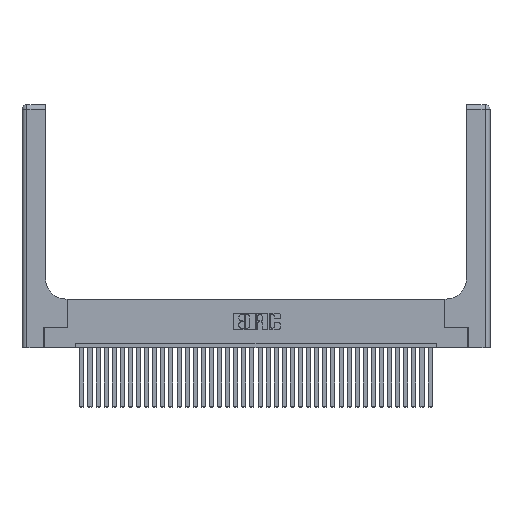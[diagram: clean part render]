
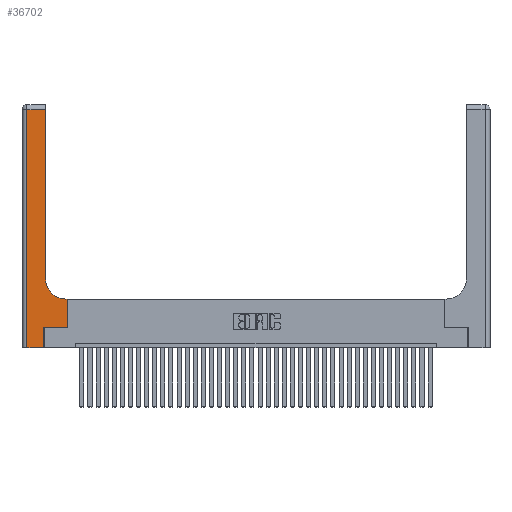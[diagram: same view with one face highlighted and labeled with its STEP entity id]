
A CAD part, top view. The second image highlights one B-rep face of the part: STEP entity #36702.
In plain terms, the highlighted planar face has unit normal (0, 0, 1).
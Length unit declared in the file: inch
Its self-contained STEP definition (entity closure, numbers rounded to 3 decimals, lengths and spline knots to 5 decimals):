
#1212 = EDGE_CURVE ( 'NONE', #21255, #14753, #31797, .T. ) ;
#1255 = ORIENTED_EDGE ( 'NONE', *, *, #15979, .T. ) ;
#1285 = VECTOR ( 'NONE', #25667, 39.37008 ) ;
#1435 = AXIS2_PLACEMENT_3D ( 'NONE', #23984, #33215, #32696 ) ;
#1765 = CARTESIAN_POINT ( 'NONE',  ( 0.269, 0.25, 0.37 ) ) ;
#3173 = EDGE_CURVE ( 'NONE', #29049, #30460, #33925, .T. ) ;
#5158 = VECTOR ( 'NONE', #18472, 39.37008 ) ;
#5748 = EDGE_CURVE ( 'NONE', #18772, #14261, #11396, .T. ) ;
#5871 = ORIENTED_EDGE ( 'NONE', *, *, #26696, .T. ) ;
#6200 = LINE ( 'NONE', #12929, #25857 ) ;
#7233 = EDGE_CURVE ( 'NONE', #22780, #21255, #22249, .T. ) ;
#8981 = DIRECTION ( 'NONE',  ( 0., 0., -1. ) ) ;
#9967 = PLANE ( 'NONE',  #1435 ) ;
#10083 = CARTESIAN_POINT ( 'NONE',  ( 0.06, 3., 0.37 ) ) ;
#10801 = LINE ( 'NONE', #23806, #26742 ) ;
#11307 = CARTESIAN_POINT ( 'NONE',  ( 0.5585, 0.25, 0.37 ) ) ;
#11396 = LINE ( 'NONE', #31451, #1285 ) ;
#12118 = LINE ( 'NONE', #1765, #15316 ) ;
#12406 = ORIENTED_EDGE ( 'NONE', *, *, #3173, .T. ) ;
#12929 = CARTESIAN_POINT ( 'NONE',  ( 0., 0., 0.37 ) ) ;
#14261 = VERTEX_POINT ( 'NONE', #28065 ) ;
#14459 = VECTOR ( 'NONE', #26852, 39.37008 ) ;
#14557 = VERTEX_POINT ( 'NONE', #18210 ) ;
#14695 = ORIENTED_EDGE ( 'NONE', *, *, #1212, .T. ) ;
#14753 = VERTEX_POINT ( 'NONE', #17318 ) ;
#15316 = VECTOR ( 'NONE', #27945, 39.37008 ) ;
#15547 = CARTESIAN_POINT ( 'NONE',  ( 0.2915, 3., 0.37 ) ) ;
#15565 = DIRECTION ( 'NONE',  ( 0., -1., 0. ) ) ;
#15979 = EDGE_CURVE ( 'NONE', #30460, #25708, #10801, .T. ) ;
#17318 = CARTESIAN_POINT ( 'NONE',  ( 0.5415, 0.6, 0.37 ) ) ;
#17319 = ORIENTED_EDGE ( 'NONE', *, *, #27669, .T. ) ;
#17400 = EDGE_CURVE ( 'NONE', #14557, #18772, #6200, .T. ) ;
#18210 = CARTESIAN_POINT ( 'NONE',  ( 0.06, 0., 0.37 ) ) ;
#18472 = DIRECTION ( 'NONE',  ( 0., 1., 0. ) ) ;
#18548 = ORIENTED_EDGE ( 'NONE', *, *, #32583, .T. ) ;
#18772 = VERTEX_POINT ( 'NONE', #31215 ) ;
#19516 = CARTESIAN_POINT ( 'NONE',  ( 0.2915, 2.94, 0.37 ) ) ;
#20803 = CARTESIAN_POINT ( 'NONE',  ( 0.5585, 0.6, 0.37 ) ) ;
#21255 = VERTEX_POINT ( 'NONE', #20803 ) ;
#21259 = ORIENTED_EDGE ( 'NONE', *, *, #5748, .T. ) ;
#22249 = LINE ( 'NONE', #11307, #14459 ) ;
#22253 = VECTOR ( 'NONE', #15565, 39.37008 ) ;
#22780 = VERTEX_POINT ( 'NONE', #28718 ) ;
#23418 = DIRECTION ( 'NONE',  ( 1., 0., 0. ) ) ;
#23622 = CIRCLE ( 'NONE', #24887, 0.25 ) ;
#23806 = CARTESIAN_POINT ( 'NONE',  ( 0., 2.94, 0.37 ) ) ;
#23984 = CARTESIAN_POINT ( 'NONE',  ( 0., 3., 0.37 ) ) ;
#24317 = EDGE_LOOP ( 'NONE', ( #12406, #1255, #18548, #34816, #21259, #17319, #30059, #14695, #5871 ) ) ;
#24887 = AXIS2_PLACEMENT_3D ( 'NONE', #32590, #8981, #23418 ) ;
#25412 = CARTESIAN_POINT ( 'NONE',  ( 0.06, 2.94, 0.37 ) ) ;
#25667 = DIRECTION ( 'NONE',  ( 0., 1., 0. ) ) ;
#25708 = VERTEX_POINT ( 'NONE', #25412 ) ;
#25857 = VECTOR ( 'NONE', #36681, 39.37008 ) ;
#26696 = EDGE_CURVE ( 'NONE', #14753, #29049, #23622, .T. ) ;
#26742 = VECTOR ( 'NONE', #29461, 39.37008 ) ;
#26852 = DIRECTION ( 'NONE',  ( 0., 1., 0. ) ) ;
#27669 = EDGE_CURVE ( 'NONE', #14261, #22780, #12118, .T. ) ;
#27945 = DIRECTION ( 'NONE',  ( 1., 0., 0. ) ) ;
#28065 = CARTESIAN_POINT ( 'NONE',  ( 0.269, 0.25, 0.37 ) ) ;
#28672 = CARTESIAN_POINT ( 'NONE',  ( 0.2915, 0.6, 0.37 ) ) ;
#28718 = CARTESIAN_POINT ( 'NONE',  ( 0.5585, 0.25, 0.37 ) ) ;
#29049 = VERTEX_POINT ( 'NONE', #29545 ) ;
#29461 = DIRECTION ( 'NONE',  ( -1., 0., 0. ) ) ;
#29545 = CARTESIAN_POINT ( 'NONE',  ( 0.2915, 0.85, 0.37 ) ) ;
#30015 = LINE ( 'NONE', #10083, #22253 ) ;
#30059 = ORIENTED_EDGE ( 'NONE', *, *, #7233, .T. ) ;
#30460 = VERTEX_POINT ( 'NONE', #19516 ) ;
#30902 = VECTOR ( 'NONE', #31273, 39.37008 ) ;
#31215 = CARTESIAN_POINT ( 'NONE',  ( 0.269, 0., 0.37 ) ) ;
#31273 = DIRECTION ( 'NONE',  ( -1., 0., 0. ) ) ;
#31451 = CARTESIAN_POINT ( 'NONE',  ( 0.269, 0., 0.37 ) ) ;
#31797 = LINE ( 'NONE', #28672, #30902 ) ;
#32341 = FACE_OUTER_BOUND ( 'NONE', #24317, .T. ) ;
#32583 = EDGE_CURVE ( 'NONE', #25708, #14557, #30015, .T. ) ;
#32590 = CARTESIAN_POINT ( 'NONE',  ( 0.5415, 0.85, 0.37 ) ) ;
#32696 = DIRECTION ( 'NONE',  ( -1., 0., 0. ) ) ;
#33215 = DIRECTION ( 'NONE',  ( 0., 0., -1. ) ) ;
#33925 = LINE ( 'NONE', #15547, #5158 ) ;
#34816 = ORIENTED_EDGE ( 'NONE', *, *, #17400, .T. ) ;
#36681 = DIRECTION ( 'NONE',  ( 1., 0., 0. ) ) ;
#36702 = ADVANCED_FACE ( 'NONE', ( #32341 ), #9967, .F. ) ;
